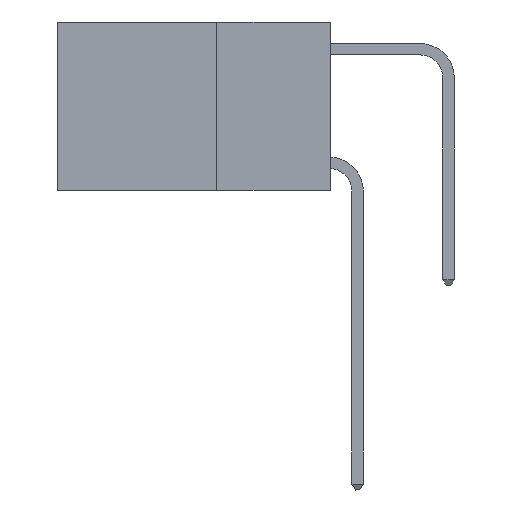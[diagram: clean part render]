
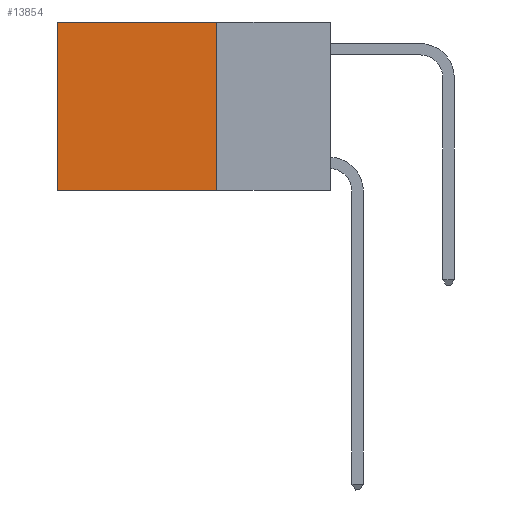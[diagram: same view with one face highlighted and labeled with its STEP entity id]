
A CAD part, left-side view. The second image highlights one B-rep face of the part: STEP entity #13854.
In plain terms, the highlighted planar face has unit normal (-1, 0, 0).
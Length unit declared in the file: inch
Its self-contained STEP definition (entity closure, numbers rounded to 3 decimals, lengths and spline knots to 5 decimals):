
#69 = ORIENTED_EDGE ( 'NONE', *, *, #8479, .T. ) ;
#425 = VECTOR ( 'NONE', #1549, 39.37008 ) ;
#744 = EDGE_CURVE ( 'NONE', #3920, #6284, #13836, .T. ) ;
#857 = EDGE_CURVE ( 'NONE', #13152, #3920, #3249, .T. ) ;
#869 = DIRECTION ( 'NONE',  ( 0., 1., 0. ) ) ;
#1060 = PLANE ( 'NONE',  #1736 ) ;
#1458 = CARTESIAN_POINT ( 'NONE',  ( 0.2625, 0.6, 0. ) ) ;
#1479 = CARTESIAN_POINT ( 'NONE',  ( 0.2625, 0.25, 0. ) ) ;
#1549 = DIRECTION ( 'NONE',  ( 0., 1., 0. ) ) ;
#1736 = AXIS2_PLACEMENT_3D ( 'NONE', #16040, #7904, #5378 ) ;
#3249 = LINE ( 'NONE', #11169, #7065 ) ;
#3920 = VERTEX_POINT ( 'NONE', #17491 ) ;
#4344 = DIRECTION ( 'NONE',  ( 0., 0., -1. ) ) ;
#5378 = DIRECTION ( 'NONE',  ( 0., 0., -1. ) ) ;
#6284 = VERTEX_POINT ( 'NONE', #11355 ) ;
#6520 = LINE ( 'NONE', #8056, #16822 ) ;
#6550 = ORIENTED_EDGE ( 'NONE', *, *, #857, .F. ) ;
#7065 = VECTOR ( 'NONE', #4344, 39.37008 ) ;
#7904 = DIRECTION ( 'NONE',  ( 1., 0., 0. ) ) ;
#8056 = CARTESIAN_POINT ( 'NONE',  ( 0.2625, 0.6, 0. ) ) ;
#8114 = ORIENTED_EDGE ( 'NONE', *, *, #744, .F. ) ;
#8479 = EDGE_CURVE ( 'NONE', #13548, #6284, #6520, .T. ) ;
#9165 = CARTESIAN_POINT ( 'NONE',  ( 0.2625, 0.25, 0. ) ) ;
#11169 = CARTESIAN_POINT ( 'NONE',  ( 0.2625, 0.25, 0. ) ) ;
#11355 = CARTESIAN_POINT ( 'NONE',  ( 0.2625, 0.6, -0.37 ) ) ;
#13152 = VERTEX_POINT ( 'NONE', #1479 ) ;
#13524 = FACE_OUTER_BOUND ( 'NONE', #14693, .T. ) ;
#13548 = VERTEX_POINT ( 'NONE', #1458 ) ;
#13836 = LINE ( 'NONE', #16617, #425 ) ;
#13854 = ADVANCED_FACE ( 'NONE', ( #13524 ), #1060, .F. ) ;
#14498 = LINE ( 'NONE', #9165, #14910 ) ;
#14693 = EDGE_LOOP ( 'NONE', ( #69, #8114, #6550, #15105 ) ) ;
#14910 = VECTOR ( 'NONE', #869, 39.37008 ) ;
#15105 = ORIENTED_EDGE ( 'NONE', *, *, #15765, .T. ) ;
#15765 = EDGE_CURVE ( 'NONE', #13152, #13548, #14498, .T. ) ;
#16040 = CARTESIAN_POINT ( 'NONE',  ( 0.2625, 0.25, 0. ) ) ;
#16617 = CARTESIAN_POINT ( 'NONE',  ( 0.2625, 0.25, -0.37 ) ) ;
#16822 = VECTOR ( 'NONE', #17447, 39.37008 ) ;
#17447 = DIRECTION ( 'NONE',  ( 0., 0., -1. ) ) ;
#17491 = CARTESIAN_POINT ( 'NONE',  ( 0.2625, 0.25, -0.37 ) ) ;
